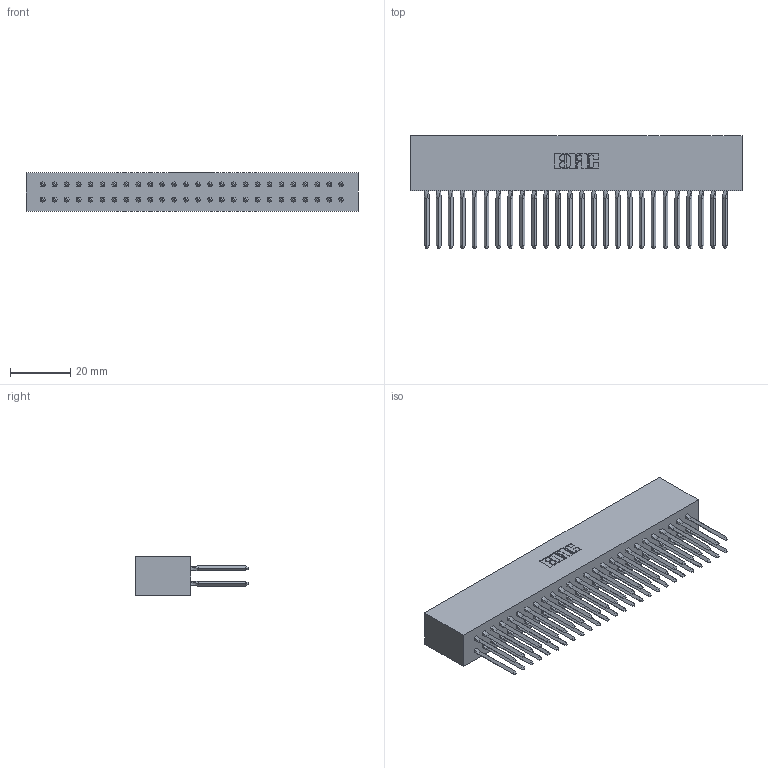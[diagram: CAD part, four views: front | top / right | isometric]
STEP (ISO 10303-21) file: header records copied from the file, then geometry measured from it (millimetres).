
FILE_DESCRIPTION (( 'STEP AP203' ), '1' );
FILE_NAME ('317-052-542-801.STEP', '2020-02-28T03:31:20', ( '' ), ( '' ), 'SwSTEP 2.0', 'SolidWorks 2016', '' );
FILE_SCHEMA (( 'CONFIG_CONTROL_DESIGN' ));
Length unit declared in the file: inch
Products named in the file (3): 317-290-003_542; 317 Part_Lugless; 317-052-542-801
Assembly tree (53 placements, depth 2):
  317-052-542-801
    317 Part_Lugless
    317-290-003_542  x52
Bounding box: 110.24 x 37.34 x 12.7 mm (x, y, z)
Volume: 19275.4 mm3; surface area: 26467.6 mm2
Topology: 53 solids, 53 shells, 3054 faces, 8559 edges, 5462 vertices
Faces by surface type: plane 2442, cylinder 404, bspline 208
Entity records: 38423 total; most frequent: CARTESIAN_POINT 6949, ORIENTED_EDGE 6612, DIRECTION 5582, EDGE_CURVE 3306, LINE 3144, VECTOR 3144, VERTEX_POINT 2198, AXIS2_PLACEMENT_3D 1219
